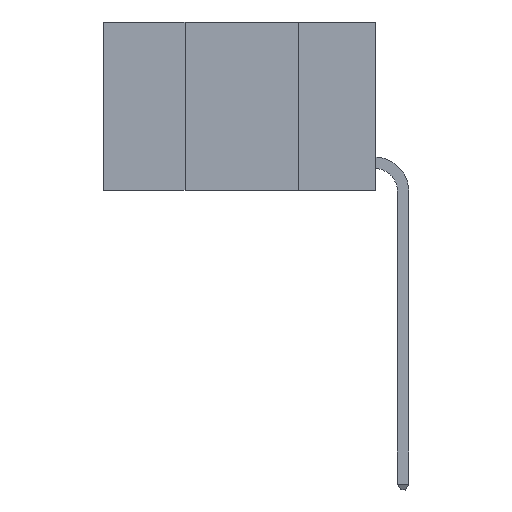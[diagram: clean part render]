
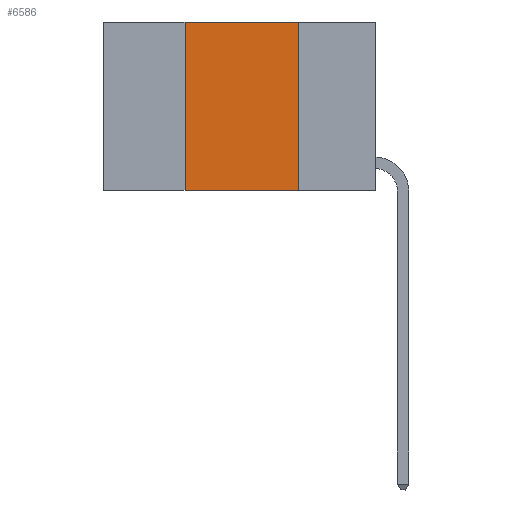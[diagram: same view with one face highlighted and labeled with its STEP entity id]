
A CAD part, left-side view. The second image highlights one B-rep face of the part: STEP entity #6586.
In plain terms, the highlighted planar face has unit normal (-1, 0, 0).
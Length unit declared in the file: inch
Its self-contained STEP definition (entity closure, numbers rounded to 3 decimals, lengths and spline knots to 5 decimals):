
#185 = LINE ( 'NONE', #16731, #7959 ) ;
#2485 = DIRECTION ( 'NONE',  ( 0., -1., 0. ) ) ;
#2800 = VERTEX_POINT ( 'NONE', #18164 ) ;
#2942 = DIRECTION ( 'NONE',  ( 0., 0., 1. ) ) ;
#3068 = PLANE ( 'NONE',  #12165 ) ;
#3732 = EDGE_CURVE ( 'NONE', #7253, #14547, #11559, .T. ) ;
#4669 = VECTOR ( 'NONE', #2485, 39.37008 ) ;
#6586 = ADVANCED_FACE ( 'NONE', ( #7846 ), #3068, .F. ) ;
#7253 = VERTEX_POINT ( 'NONE', #13832 ) ;
#7726 = DIRECTION ( 'NONE',  ( 1., 0., 0. ) ) ;
#7846 = FACE_OUTER_BOUND ( 'NONE', #10158, .T. ) ;
#7959 = VECTOR ( 'NONE', #10675, 39.37008 ) ;
#8247 = VECTOR ( 'NONE', #2942, 39.37008 ) ;
#8335 = EDGE_CURVE ( 'NONE', #7253, #8770, #16380, .T. ) ;
#8452 = CARTESIAN_POINT ( 'NONE',  ( 0., 0.42, 0. ) ) ;
#8558 = DIRECTION ( 'NONE',  ( 0., -1., 0. ) ) ;
#8770 = VERTEX_POINT ( 'NONE', #8452 ) ;
#10158 = EDGE_LOOP ( 'NONE', ( #17284, #17272, #10615, #14856 ) ) ;
#10261 = CARTESIAN_POINT ( 'NONE',  ( 0., 0.6, 0. ) ) ;
#10615 = ORIENTED_EDGE ( 'NONE', *, *, #8335, .F. ) ;
#10635 = CARTESIAN_POINT ( 'NONE',  ( 0., 0.42, 0. ) ) ;
#10675 = DIRECTION ( 'NONE',  ( 0., 0., -1. ) ) ;
#11559 = LINE ( 'NONE', #14610, #15097 ) ;
#12165 = AXIS2_PLACEMENT_3D ( 'NONE', #16873, #7726, #18434 ) ;
#13832 = CARTESIAN_POINT ( 'NONE',  ( 0., 0.42, -0.37 ) ) ;
#13861 = EDGE_CURVE ( 'NONE', #2800, #14547, #185, .T. ) ;
#13877 = CARTESIAN_POINT ( 'NONE',  ( 0., 0.17, -0.37 ) ) ;
#14547 = VERTEX_POINT ( 'NONE', #13877 ) ;
#14610 = CARTESIAN_POINT ( 'NONE',  ( 0., 0.6, -0.37 ) ) ;
#14856 = ORIENTED_EDGE ( 'NONE', *, *, #3732, .T. ) ;
#15097 = VECTOR ( 'NONE', #8558, 39.37008 ) ;
#16380 = LINE ( 'NONE', #10635, #8247 ) ;
#16411 = LINE ( 'NONE', #10261, #4669 ) ;
#16731 = CARTESIAN_POINT ( 'NONE',  ( 0., 0.17, 0. ) ) ;
#16873 = CARTESIAN_POINT ( 'NONE',  ( 0., 0.6, 0. ) ) ;
#17272 = ORIENTED_EDGE ( 'NONE', *, *, #18195, .F. ) ;
#17284 = ORIENTED_EDGE ( 'NONE', *, *, #13861, .F. ) ;
#18164 = CARTESIAN_POINT ( 'NONE',  ( 0., 0.17, 0. ) ) ;
#18195 = EDGE_CURVE ( 'NONE', #8770, #2800, #16411, .T. ) ;
#18434 = DIRECTION ( 'NONE',  ( 0., 0., -1. ) ) ;
